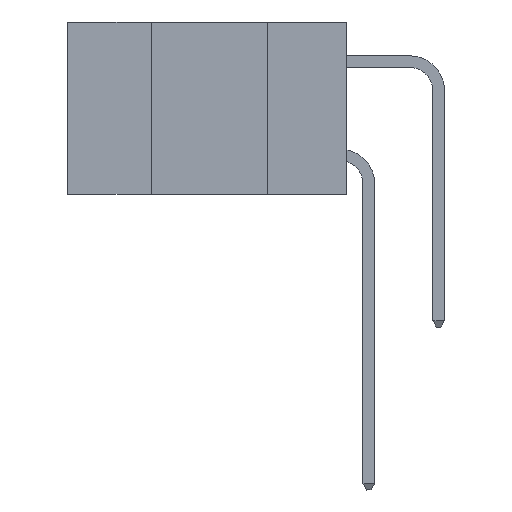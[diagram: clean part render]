
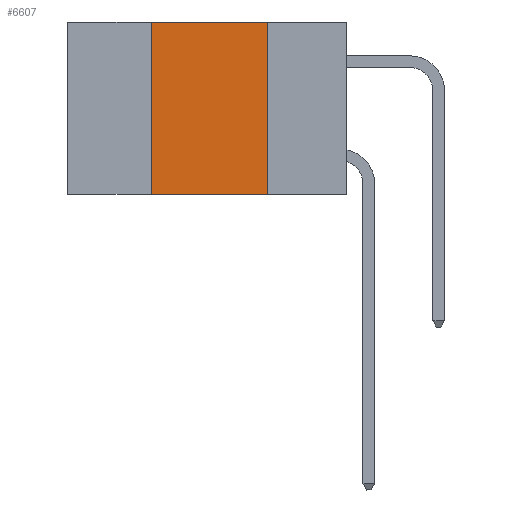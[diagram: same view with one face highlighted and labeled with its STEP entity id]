
A CAD part, left-side view. The second image highlights one B-rep face of the part: STEP entity #6607.
In plain terms, the highlighted planar face has unit normal (-1, 0, 0).
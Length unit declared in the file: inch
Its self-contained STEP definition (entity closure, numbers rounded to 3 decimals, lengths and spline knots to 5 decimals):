
#518 = ORIENTED_EDGE ( 'NONE', *, *, #19661, .F. ) ;
#814 = ORIENTED_EDGE ( 'NONE', *, *, #5591, .T. ) ;
#1368 = DIRECTION ( 'NONE',  ( 0., 0., -1. ) ) ;
#1600 = DIRECTION ( 'NONE',  ( 0., 0., 1. ) ) ;
#1682 = VECTOR ( 'NONE', #17635, 39.37008 ) ;
#2218 = CARTESIAN_POINT ( 'NONE',  ( 0., 0.42, 0. ) ) ;
#2294 = LINE ( 'NONE', #12097, #18468 ) ;
#2710 = EDGE_CURVE ( 'NONE', #11509, #15000, #20048, .T. ) ;
#4163 = VERTEX_POINT ( 'NONE', #2218 ) ;
#4671 = VECTOR ( 'NONE', #1600, 39.37008 ) ;
#5591 = EDGE_CURVE ( 'NONE', #5855, #15000, #2294, .T. ) ;
#5855 = VERTEX_POINT ( 'NONE', #14199 ) ;
#6209 = AXIS2_PLACEMENT_3D ( 'NONE', #13907, #10858, #1368 ) ;
#6607 = ADVANCED_FACE ( 'NONE', ( #16269 ), #20086, .F. ) ;
#8148 = DIRECTION ( 'NONE',  ( 0., 0., -1. ) ) ;
#9671 = EDGE_CURVE ( 'NONE', #5855, #4163, #17103, .T. ) ;
#10858 = DIRECTION ( 'NONE',  ( 1., 0., 0. ) ) ;
#11231 = CARTESIAN_POINT ( 'NONE',  ( 0., 0.17, -0.37 ) ) ;
#11509 = VERTEX_POINT ( 'NONE', #20230 ) ;
#12097 = CARTESIAN_POINT ( 'NONE',  ( 0., 0.6, -0.37 ) ) ;
#12201 = ORIENTED_EDGE ( 'NONE', *, *, #2710, .F. ) ;
#12654 = CARTESIAN_POINT ( 'NONE',  ( 0., 0.17, 0. ) ) ;
#13907 = CARTESIAN_POINT ( 'NONE',  ( 0., 0.6, 0. ) ) ;
#14199 = CARTESIAN_POINT ( 'NONE',  ( 0., 0.42, -0.37 ) ) ;
#14670 = EDGE_LOOP ( 'NONE', ( #12201, #518, #15594, #814 ) ) ;
#15000 = VERTEX_POINT ( 'NONE', #11231 ) ;
#15594 = ORIENTED_EDGE ( 'NONE', *, *, #9671, .F. ) ;
#15722 = CARTESIAN_POINT ( 'NONE',  ( 0., 0.42, 0. ) ) ;
#15957 = VECTOR ( 'NONE', #8148, 39.37008 ) ;
#16062 = CARTESIAN_POINT ( 'NONE',  ( 0., 0.6, 0. ) ) ;
#16269 = FACE_OUTER_BOUND ( 'NONE', #14670, .T. ) ;
#17103 = LINE ( 'NONE', #15722, #4671 ) ;
#17635 = DIRECTION ( 'NONE',  ( 0., -1., 0. ) ) ;
#18338 = LINE ( 'NONE', #16062, #1682 ) ;
#18468 = VECTOR ( 'NONE', #19788, 39.37008 ) ;
#19661 = EDGE_CURVE ( 'NONE', #4163, #11509, #18338, .T. ) ;
#19788 = DIRECTION ( 'NONE',  ( 0., -1., 0. ) ) ;
#20048 = LINE ( 'NONE', #12654, #15957 ) ;
#20086 = PLANE ( 'NONE',  #6209 ) ;
#20230 = CARTESIAN_POINT ( 'NONE',  ( 0., 0.17, 0. ) ) ;
